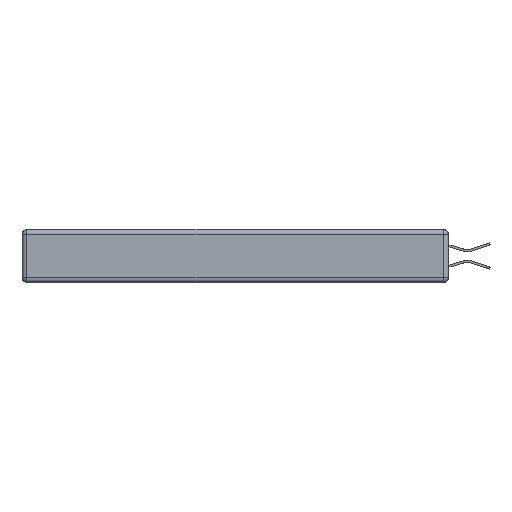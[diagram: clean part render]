
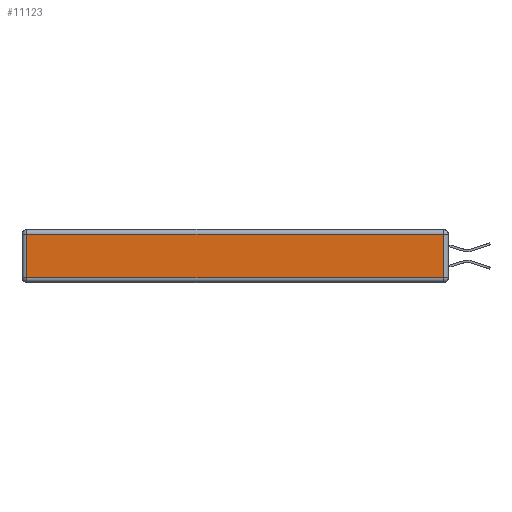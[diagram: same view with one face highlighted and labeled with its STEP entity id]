
A CAD part, left-side view. The second image highlights one B-rep face of the part: STEP entity #11123.
In plain terms, the highlighted planar face has unit normal (-1, 0, 0).
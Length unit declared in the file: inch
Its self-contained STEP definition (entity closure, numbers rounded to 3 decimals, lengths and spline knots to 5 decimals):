
#207 = CARTESIAN_POINT ( 'NONE',  ( 0., 2.75, -0.03 ) ) ;
#747 = ORIENTED_EDGE ( 'NONE', *, *, #9505, .T. ) ;
#1488 = AXIS2_PLACEMENT_3D ( 'NONE', #13122, #11108, #7257 ) ;
#2861 = LINE ( 'NONE', #16442, #19360 ) ;
#4058 = DIRECTION ( 'NONE',  ( 0., 1., 0. ) ) ;
#4950 = LINE ( 'NONE', #5346, #14564 ) ;
#4959 = ORIENTED_EDGE ( 'NONE', *, *, #12889, .T. ) ;
#4987 = VERTEX_POINT ( 'NONE', #5188 ) ;
#5188 = CARTESIAN_POINT ( 'NONE',  ( 0., 2.72, -0.03 ) ) ;
#5346 = CARTESIAN_POINT ( 'NONE',  ( 0., 0., -0.313 ) ) ;
#5620 = VERTEX_POINT ( 'NONE', #9544 ) ;
#5726 = CARTESIAN_POINT ( 'NONE',  ( 0., 0.03, -0.343 ) ) ;
#6488 = VECTOR ( 'NONE', #4058, 39.37008 ) ;
#7229 = DIRECTION ( 'NONE',  ( 0., 0., -1. ) ) ;
#7257 = DIRECTION ( 'NONE',  ( 0., 0., 1. ) ) ;
#7297 = ORIENTED_EDGE ( 'NONE', *, *, #16945, .T. ) ;
#7577 = DIRECTION ( 'NONE',  ( 0., 0., 1. ) ) ;
#8486 = CARTESIAN_POINT ( 'NONE',  ( 0., 0.03, -0.03 ) ) ;
#9187 = DIRECTION ( 'NONE',  ( 0., -1., 0. ) ) ;
#9505 = EDGE_CURVE ( 'NONE', #15038, #4987, #19951, .T. ) ;
#9544 = CARTESIAN_POINT ( 'NONE',  ( 0., 2.72, -0.313 ) ) ;
#10996 = EDGE_LOOP ( 'NONE', ( #24713, #4959, #747, #7297 ) ) ;
#11108 = DIRECTION ( 'NONE',  ( -1., 0., 0. ) ) ;
#11123 = ADVANCED_FACE ( 'NONE', ( #12476 ), #12934, .T. ) ;
#11756 = EDGE_CURVE ( 'NONE', #5620, #19700, #4950, .T. ) ;
#12476 = FACE_OUTER_BOUND ( 'NONE', #10996, .T. ) ;
#12694 = LINE ( 'NONE', #5726, #14812 ) ;
#12889 = EDGE_CURVE ( 'NONE', #19700, #15038, #12694, .T. ) ;
#12934 = PLANE ( 'NONE',  #1488 ) ;
#13122 = CARTESIAN_POINT ( 'NONE',  ( 0., 0., -0.343 ) ) ;
#14564 = VECTOR ( 'NONE', #9187, 39.37008 ) ;
#14812 = VECTOR ( 'NONE', #7577, 39.37008 ) ;
#15038 = VERTEX_POINT ( 'NONE', #8486 ) ;
#16442 = CARTESIAN_POINT ( 'NONE',  ( 0., 2.72, -0.343 ) ) ;
#16945 = EDGE_CURVE ( 'NONE', #4987, #5620, #2861, .T. ) ;
#19360 = VECTOR ( 'NONE', #7229, 39.37008 ) ;
#19700 = VERTEX_POINT ( 'NONE', #23671 ) ;
#19951 = LINE ( 'NONE', #207, #6488 ) ;
#23671 = CARTESIAN_POINT ( 'NONE',  ( 0., 0.03, -0.313 ) ) ;
#24713 = ORIENTED_EDGE ( 'NONE', *, *, #11756, .T. ) ;
